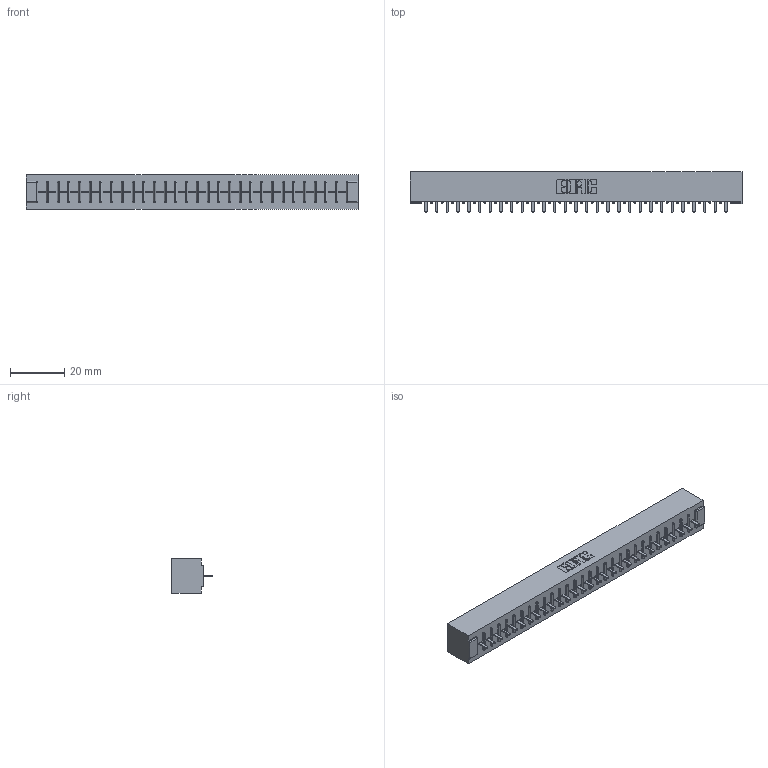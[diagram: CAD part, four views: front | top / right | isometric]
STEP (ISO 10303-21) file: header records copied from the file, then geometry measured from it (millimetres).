
FILE_DESCRIPTION (( 'STEP AP203' ), '1' );
FILE_NAME ('356-029-421-101.STEP', '2020-09-23T19:07:49', ( '' ), ( '' ), 'SwSTEP 2.0', 'SolidWorks 2020', '' );
FILE_SCHEMA (( 'CONFIG_CONTROL_DESIGN' ));
Length unit declared in the file: inch
Products named in the file (3): 356-029-421-101; 306-290-001_121; 306 Part_No Mounting
Assembly tree (30 placements, depth 2):
  356-029-421-101
    306 Part_No Mounting
    306-290-001_121  x29
Bounding box: 122.78 x 14.88 x 12.7 mm (x, y, z)
Volume: 13999 mm3; surface area: 14162.3 mm2
Topology: 30 solids, 30 shells, 2138 faces, 6005 edges, 3846 vertices
Faces by surface type: plane 1427, cylinder 595, sphere 116
Entity records: 28406 total; most frequent: CARTESIAN_POINT 4766, ORIENTED_EDGE 4722, DIRECTION 4701, EDGE_CURVE 2361, VECTOR 1843, LINE 1843, VERTEX_POINT 1494, AXIS2_PLACEMENT_3D 1429
